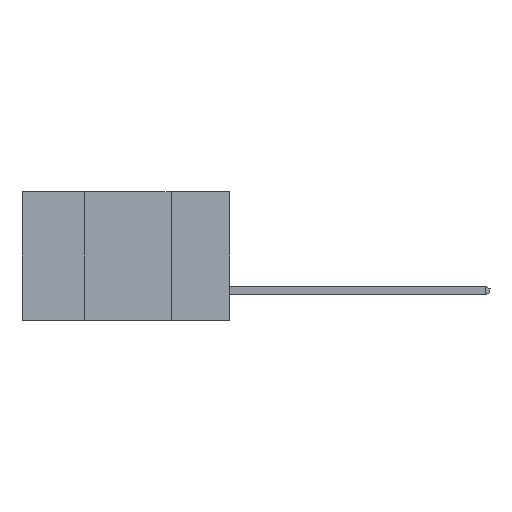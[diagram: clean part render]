
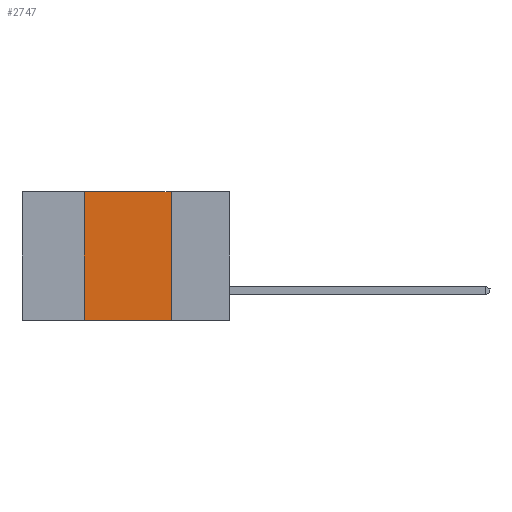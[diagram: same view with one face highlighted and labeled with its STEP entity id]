
A CAD part, left-side view. The second image highlights one B-rep face of the part: STEP entity #2747.
In plain terms, the highlighted planar face has unit normal (-1, 0, 0).
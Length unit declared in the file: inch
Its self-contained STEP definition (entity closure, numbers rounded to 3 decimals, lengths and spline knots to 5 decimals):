
#556 = VERTEX_POINT ( 'NONE', #6077 ) ;
#761 = LINE ( 'NONE', #2353, #8649 ) ;
#771 = FACE_OUTER_BOUND ( 'NONE', #9562, .T. ) ;
#1171 = EDGE_CURVE ( 'NONE', #4928, #556, #761, .T. ) ;
#2353 = CARTESIAN_POINT ( 'NONE',  ( 0., 0.17, -0.37 ) ) ;
#2747 = ADVANCED_FACE ( 'NONE', ( #771 ), #3155, .F. ) ;
#3155 = PLANE ( 'NONE',  #9072 ) ;
#3328 = DIRECTION ( 'NONE',  ( 1., 0., 0. ) ) ;
#3571 = EDGE_CURVE ( 'NONE', #3813, #556, #5699, .T. ) ;
#3813 = VERTEX_POINT ( 'NONE', #4528 ) ;
#3934 = VECTOR ( 'NONE', #4068, 39.37008 ) ;
#3955 = ORIENTED_EDGE ( 'NONE', *, *, #8096, .F. ) ;
#3992 = CARTESIAN_POINT ( 'NONE',  ( 0., 0.6, 0. ) ) ;
#4068 = DIRECTION ( 'NONE',  ( 0., -1., 0. ) ) ;
#4521 = ORIENTED_EDGE ( 'NONE', *, *, #3571, .T. ) ;
#4528 = CARTESIAN_POINT ( 'NONE',  ( 0., 0.42, -0.37 ) ) ;
#4608 = ORIENTED_EDGE ( 'NONE', *, *, #1171, .F. ) ;
#4841 = CARTESIAN_POINT ( 'NONE',  ( 0., 0.6, -0.37 ) ) ;
#4928 = VERTEX_POINT ( 'NONE', #7833 ) ;
#4933 = CARTESIAN_POINT ( 'NONE',  ( 0., 0.6, 0. ) ) ;
#5063 = CARTESIAN_POINT ( 'NONE',  ( 0., 0.42, -0.37 ) ) ;
#5173 = EDGE_CURVE ( 'NONE', #10015, #4928, #8486, .T. ) ;
#5699 = LINE ( 'NONE', #4841, #3934 ) ;
#5929 = DIRECTION ( 'NONE',  ( 0., 0., 1. ) ) ;
#6077 = CARTESIAN_POINT ( 'NONE',  ( 0., 0.17, -0.37 ) ) ;
#6816 = DIRECTION ( 'NONE',  ( 0., 0., -1. ) ) ;
#7803 = DIRECTION ( 'NONE',  ( 0., 0., -1. ) ) ;
#7833 = CARTESIAN_POINT ( 'NONE',  ( 0., 0.17, 0. ) ) ;
#7961 = CARTESIAN_POINT ( 'NONE',  ( 0., 0.42, 0. ) ) ;
#8096 = EDGE_CURVE ( 'NONE', #3813, #10015, #11258, .T. ) ;
#8486 = LINE ( 'NONE', #3992, #10591 ) ;
#8649 = VECTOR ( 'NONE', #6816, 39.37008 ) ;
#9072 = AXIS2_PLACEMENT_3D ( 'NONE', #4933, #3328, #7803 ) ;
#9562 = EDGE_LOOP ( 'NONE', ( #4608, #9984, #3955, #4521 ) ) ;
#9984 = ORIENTED_EDGE ( 'NONE', *, *, #5173, .F. ) ;
#10015 = VERTEX_POINT ( 'NONE', #7961 ) ;
#10591 = VECTOR ( 'NONE', #10704, 39.37008 ) ;
#10704 = DIRECTION ( 'NONE',  ( 0., -1., 0. ) ) ;
#11199 = VECTOR ( 'NONE', #5929, 39.37008 ) ;
#11258 = LINE ( 'NONE', #5063, #11199 ) ;
